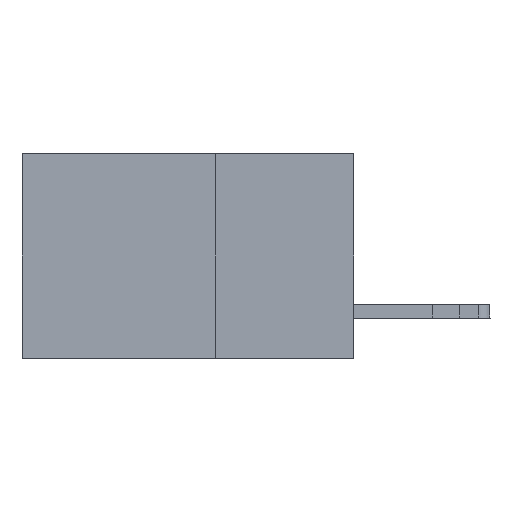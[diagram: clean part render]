
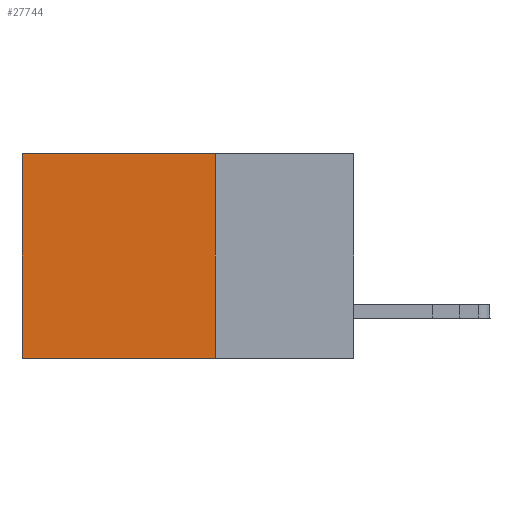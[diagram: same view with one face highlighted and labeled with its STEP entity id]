
A CAD part, left-side view. The second image highlights one B-rep face of the part: STEP entity #27744.
In plain terms, the highlighted planar face has unit normal (-1, 0, 0).
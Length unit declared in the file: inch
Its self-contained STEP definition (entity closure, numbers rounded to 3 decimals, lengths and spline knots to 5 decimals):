
#310 = VERTEX_POINT ( 'NONE', #35705 ) ;
#2399 = VECTOR ( 'NONE', #27598, 39.37008 ) ;
#3527 = VERTEX_POINT ( 'NONE', #31479 ) ;
#3781 = VECTOR ( 'NONE', #15924, 39.37008 ) ;
#6031 = LINE ( 'NONE', #7436, #19891 ) ;
#7004 = VERTEX_POINT ( 'NONE', #31119 ) ;
#7436 = CARTESIAN_POINT ( 'NONE',  ( 0.2875, 0.25, 0. ) ) ;
#7532 = VERTEX_POINT ( 'NONE', #21787 ) ;
#7850 = PLANE ( 'NONE',  #31069 ) ;
#9971 = CARTESIAN_POINT ( 'NONE',  ( 0.2875, 0.25, -0.37 ) ) ;
#10847 = DIRECTION ( 'NONE',  ( 0., 0., -1. ) ) ;
#13391 = DIRECTION ( 'NONE',  ( 0., 0., -1. ) ) ;
#14106 = FACE_OUTER_BOUND ( 'NONE', #33735, .T. ) ;
#15924 = DIRECTION ( 'NONE',  ( 0., 0., -1. ) ) ;
#16997 = VECTOR ( 'NONE', #19802, 39.37008 ) ;
#17723 = EDGE_CURVE ( 'NONE', #7004, #7532, #33871, .T. ) ;
#19385 = ORIENTED_EDGE ( 'NONE', *, *, #28869, .T. ) ;
#19802 = DIRECTION ( 'NONE',  ( 0., 1., 0. ) ) ;
#19891 = VECTOR ( 'NONE', #13391, 39.37008 ) ;
#21787 = CARTESIAN_POINT ( 'NONE',  ( 0.2875, 0.6, -0.37 ) ) ;
#22500 = EDGE_CURVE ( 'NONE', #3527, #7004, #6031, .T. ) ;
#22568 = CARTESIAN_POINT ( 'NONE',  ( 0.2875, 0.25, 0. ) ) ;
#24017 = ORIENTED_EDGE ( 'NONE', *, *, #17723, .F. ) ;
#24753 = LINE ( 'NONE', #37471, #16997 ) ;
#24919 = EDGE_CURVE ( 'NONE', #3527, #310, #24753, .T. ) ;
#27598 = DIRECTION ( 'NONE',  ( 0., 1., 0. ) ) ;
#27744 = ADVANCED_FACE ( 'NONE', ( #14106 ), #7850, .F. ) ;
#28472 = DIRECTION ( 'NONE',  ( 1., 0., 0. ) ) ;
#28869 = EDGE_CURVE ( 'NONE', #310, #7532, #34289, .T. ) ;
#29595 = ORIENTED_EDGE ( 'NONE', *, *, #24919, .T. ) ;
#29948 = ORIENTED_EDGE ( 'NONE', *, *, #22500, .F. ) ;
#31069 = AXIS2_PLACEMENT_3D ( 'NONE', #22568, #28472, #10847 ) ;
#31119 = CARTESIAN_POINT ( 'NONE',  ( 0.2875, 0.25, -0.37 ) ) ;
#31479 = CARTESIAN_POINT ( 'NONE',  ( 0.2875, 0.25, 0. ) ) ;
#33577 = CARTESIAN_POINT ( 'NONE',  ( 0.2875, 0.6, 0. ) ) ;
#33735 = EDGE_LOOP ( 'NONE', ( #19385, #24017, #29948, #29595 ) ) ;
#33871 = LINE ( 'NONE', #9971, #2399 ) ;
#34289 = LINE ( 'NONE', #33577, #3781 ) ;
#35705 = CARTESIAN_POINT ( 'NONE',  ( 0.2875, 0.6, 0. ) ) ;
#37471 = CARTESIAN_POINT ( 'NONE',  ( 0.2875, 0.25, 0. ) ) ;
